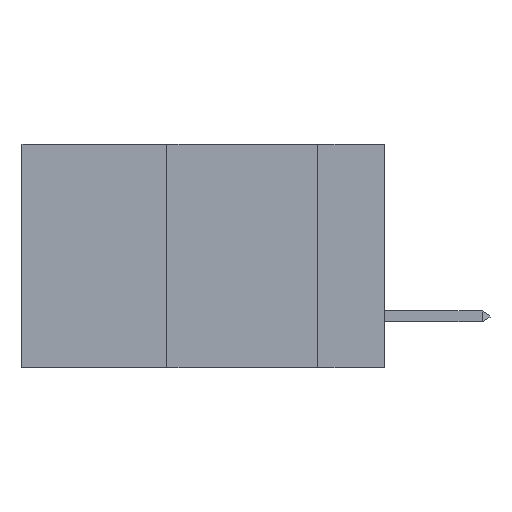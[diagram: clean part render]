
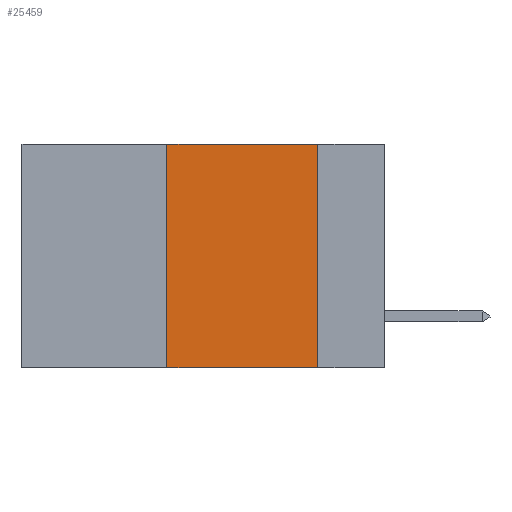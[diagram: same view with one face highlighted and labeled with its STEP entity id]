
A CAD part, left-side view. The second image highlights one B-rep face of the part: STEP entity #25459.
In plain terms, the highlighted planar face has unit normal (-1, 0, 0).
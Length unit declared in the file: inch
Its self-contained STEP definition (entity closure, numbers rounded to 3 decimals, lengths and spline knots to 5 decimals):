
#1614 = AXIS2_PLACEMENT_3D ( 'NONE', #28043, #11119, #30860 ) ;
#1993 = FACE_OUTER_BOUND ( 'NONE', #13482, .T. ) ;
#2903 = DIRECTION ( 'NONE',  ( 0., 0., -1. ) ) ;
#3188 = LINE ( 'NONE', #24364, #17486 ) ;
#3403 = CARTESIAN_POINT ( 'NONE',  ( 0., 0.6, -0.37 ) ) ;
#3727 = CARTESIAN_POINT ( 'NONE',  ( 0., 0.11, -0.37 ) ) ;
#6555 = EDGE_CURVE ( 'NONE', #11652, #12997, #36201, .T. ) ;
#8817 = VECTOR ( 'NONE', #32436, 39.37008 ) ;
#9656 = VECTOR ( 'NONE', #2903, 39.37008 ) ;
#9859 = CARTESIAN_POINT ( 'NONE',  ( 0., 0.36, 0. ) ) ;
#11119 = DIRECTION ( 'NONE',  ( 1., 0., 0. ) ) ;
#11439 = ORIENTED_EDGE ( 'NONE', *, *, #6555, .F. ) ;
#11652 = VERTEX_POINT ( 'NONE', #24244 ) ;
#12163 = CARTESIAN_POINT ( 'NONE',  ( 0., 0.11, 0. ) ) ;
#12997 = VERTEX_POINT ( 'NONE', #26912 ) ;
#13482 = EDGE_LOOP ( 'NONE', ( #21429, #34677, #11439, #25928 ) ) ;
#14054 = VECTOR ( 'NONE', #14918, 39.37008 ) ;
#14918 = DIRECTION ( 'NONE',  ( 0., -1., 0. ) ) ;
#16081 = EDGE_CURVE ( 'NONE', #12997, #25089, #3188, .T. ) ;
#17234 = LINE ( 'NONE', #31137, #9656 ) ;
#17486 = VECTOR ( 'NONE', #32738, 39.37008 ) ;
#19555 = PLANE ( 'NONE',  #1614 ) ;
#21429 = ORIENTED_EDGE ( 'NONE', *, *, #25025, .F. ) ;
#22401 = LINE ( 'NONE', #3403, #14054 ) ;
#22447 = EDGE_CURVE ( 'NONE', #11652, #23140, #22401, .T. ) ;
#23140 = VERTEX_POINT ( 'NONE', #3727 ) ;
#24244 = CARTESIAN_POINT ( 'NONE',  ( 0., 0.36, -0.37 ) ) ;
#24364 = CARTESIAN_POINT ( 'NONE',  ( 0., 0.6, 0. ) ) ;
#25025 = EDGE_CURVE ( 'NONE', #25089, #23140, #17234, .T. ) ;
#25089 = VERTEX_POINT ( 'NONE', #12163 ) ;
#25459 = ADVANCED_FACE ( 'NONE', ( #1993 ), #19555, .F. ) ;
#25928 = ORIENTED_EDGE ( 'NONE', *, *, #22447, .T. ) ;
#26912 = CARTESIAN_POINT ( 'NONE',  ( 0., 0.36, 0. ) ) ;
#28043 = CARTESIAN_POINT ( 'NONE',  ( 0., 0.6, 0. ) ) ;
#30860 = DIRECTION ( 'NONE',  ( 0., 0., -1. ) ) ;
#31137 = CARTESIAN_POINT ( 'NONE',  ( 0., 0.11, 0. ) ) ;
#32436 = DIRECTION ( 'NONE',  ( 0., 0., 1. ) ) ;
#32738 = DIRECTION ( 'NONE',  ( 0., -1., 0. ) ) ;
#34677 = ORIENTED_EDGE ( 'NONE', *, *, #16081, .F. ) ;
#36201 = LINE ( 'NONE', #9859, #8817 ) ;
